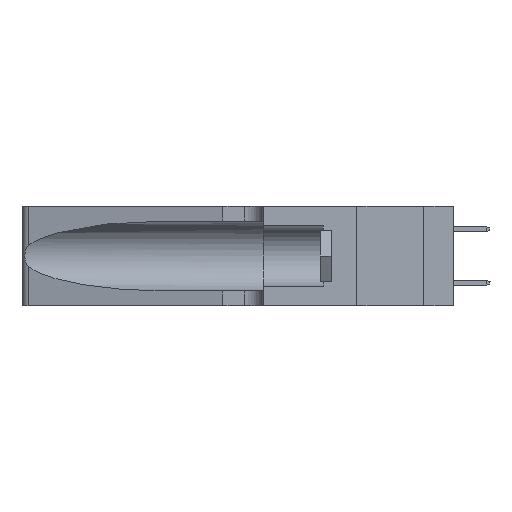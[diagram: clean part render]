
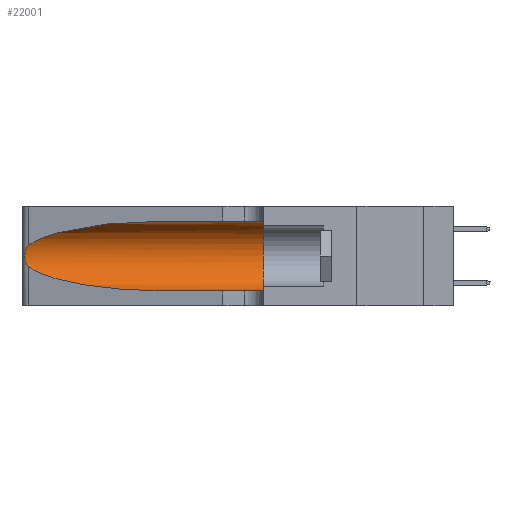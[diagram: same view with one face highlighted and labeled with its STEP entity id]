
A CAD part, left-side view. The second image highlights one B-rep face of the part: STEP entity #22001.
In plain terms, the highlighted cylindrical face has radius 3.308 mm (diameter 6.617 mm), a partial arc.
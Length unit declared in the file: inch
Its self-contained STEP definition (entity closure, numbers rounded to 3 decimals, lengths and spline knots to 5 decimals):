
#68 =( BOUNDED_CURVE ( )  B_SPLINE_CURVE ( 3, ( #24238, #24085, #4508, #12132 ),
 .UNSPECIFIED., .F., .T. ) 
 B_SPLINE_CURVE_WITH_KNOTS ( ( 4, 4 ),
 ( 3.44316, 4.71239 ),
 .UNSPECIFIED. ) 
 CURVE ( )  GEOMETRIC_REPRESENTATION_ITEM ( )  RATIONAL_B_SPLINE_CURVE ( ( 1., 0.87, 0.87, 1. ) ) 
 REPRESENTATION_ITEM ( '' )  );
#408 = VERTEX_POINT ( 'NONE', #10371 ) ;
#1938 = LINE ( 'NONE', #28831, #18233 ) ;
#2005 = CARTESIAN_POINT ( 'NONE',  ( 0.26075, 1.23896, 0.19203 ) ) ;
#2246 = EDGE_CURVE ( 'NONE', #24815, #27733, #1938, .T. ) ;
#2313 = CARTESIAN_POINT ( 'NONE',  ( 0.26075, 1.23896, 0.178 ) ) ;
#2868 = CIRCLE ( 'NONE', #19618, 0.13025 ) ;
#2886 = CARTESIAN_POINT ( 'NONE',  ( 0.2373, 1.15595, 0.28018 ) ) ;
#2993 = DIRECTION ( 'NONE',  ( 0., 1., 0. ) ) ;
#3141 =( BOUNDED_CURVE ( )  B_SPLINE_CURVE ( 3, ( #15765, #13228, #2886, #17662 ),
 .UNSPECIFIED., .F., .T. ) 
 B_SPLINE_CURVE_WITH_KNOTS ( ( 4, 4 ),
 ( 1.5708, 2.84003 ),
 .UNSPECIFIED. ) 
 CURVE ( )  GEOMETRIC_REPRESENTATION_ITEM ( )  RATIONAL_B_SPLINE_CURVE ( ( 1., 0.87, 0.87, 1. ) ) 
 REPRESENTATION_ITEM ( '' )  );
#3191 = CARTESIAN_POINT ( 'NONE',  ( 0.1305, 1.61858, 0.185 ) ) ;
#3346 = DIRECTION ( 'NONE',  ( 0., -1., 0. ) ) ;
#3574 = EDGE_LOOP ( 'NONE', ( #28299, #9650, #9836, #11445, #8035, #4098 ) ) ;
#4092 = CARTESIAN_POINT ( 'NONE',  ( 0.25787, 1.23484, 0.2124 ) ) ;
#4098 = ORIENTED_EDGE ( 'NONE', *, *, #2246, .F. ) ;
#4508 = CARTESIAN_POINT ( 'NONE',  ( 0.18966, 0.96281, 0.05475 ) ) ;
#4553 = CARTESIAN_POINT ( 'NONE',  ( 0.26017, 1.23833, 0.17102 ) ) ;
#5587 = CARTESIAN_POINT ( 'NONE',  ( 0.25487, 1.22718, 0.22369 ) ) ;
#6164 = CARTESIAN_POINT ( 'NONE',  ( 0.25487, 1.22718, 0.22369 ) ) ;
#7413 = AXIS2_PLACEMENT_3D ( 'NONE', #3191, #17329, #20341 ) ;
#7646 = CYLINDRICAL_SURFACE ( 'NONE', #7413, 0.13025 ) ;
#8035 = ORIENTED_EDGE ( 'NONE', *, *, #8123, .F. ) ;
#8123 = EDGE_CURVE ( 'NONE', #27733, #22074, #2868, .T. ) ;
#9606 = CARTESIAN_POINT ( 'NONE',  ( 0.25856, 1.23593, 0.16098 ) ) ;
#9640 = EDGE_CURVE ( 'NONE', #14535, #408, #68, .T. ) ;
#9650 = ORIENTED_EDGE ( 'NONE', *, *, #21707, .T. ) ;
#9657 = CARTESIAN_POINT ( 'NONE',  ( 0.1305, 0.35, 0.185 ) ) ;
#9673 = B_SPLINE_CURVE_WITH_KNOTS ( 'NONE', 3,
 ( #6164, #13802, #19027, #4092, #24127, #16796, #2005, #2313, #4553, #9606, #16496, #11391, #18712, #23791 ),
 .UNSPECIFIED., .F., .F.,
 ( 4, 2, 2, 2, 2, 2, 4 ),
 ( 0., 0.00027, 0.00053, 0.00107, 0.0016, 0.00187, 0.00214 ),
 .UNSPECIFIED. ) ;
#9836 = ORIENTED_EDGE ( 'NONE', *, *, #9640, .T. ) ;
#10371 = CARTESIAN_POINT ( 'NONE',  ( 0.1305, 0.72297, 0.05475 ) ) ;
#11391 = CARTESIAN_POINT ( 'NONE',  ( 0.25639, 1.23186, 0.15144 ) ) ;
#11445 = ORIENTED_EDGE ( 'NONE', *, *, #14961, .T. ) ;
#12132 = CARTESIAN_POINT ( 'NONE',  ( 0.1305, 0.72297, 0.05475 ) ) ;
#13228 = CARTESIAN_POINT ( 'NONE',  ( 0.18966, 0.96281, 0.31525 ) ) ;
#13802 = CARTESIAN_POINT ( 'NONE',  ( 0.25555, 1.22994, 0.2215 ) ) ;
#14535 = VERTEX_POINT ( 'NONE', #15484 ) ;
#14961 = EDGE_CURVE ( 'NONE', #408, #22074, #15446, .T. ) ;
#15446 = LINE ( 'NONE', #28024, #30075 ) ;
#15484 = CARTESIAN_POINT ( 'NONE',  ( 0.25487, 1.22718, 0.14631 ) ) ;
#15765 = CARTESIAN_POINT ( 'NONE',  ( 0.1305, 0.72297, 0.31525 ) ) ;
#16496 = CARTESIAN_POINT ( 'NONE',  ( 0.25789, 1.23486, 0.15765 ) ) ;
#16796 = CARTESIAN_POINT ( 'NONE',  ( 0.26018, 1.23835, 0.19895 ) ) ;
#17329 = DIRECTION ( 'NONE',  ( 0., -1., 0. ) ) ;
#17662 = CARTESIAN_POINT ( 'NONE',  ( 0.25487, 1.22718, 0.22369 ) ) ;
#18233 = VECTOR ( 'NONE', #31103, 39.37008 ) ;
#18712 = CARTESIAN_POINT ( 'NONE',  ( 0.25555, 1.22993, 0.14849 ) ) ;
#19027 = CARTESIAN_POINT ( 'NONE',  ( 0.25639, 1.23184, 0.21858 ) ) ;
#19618 = AXIS2_PLACEMENT_3D ( 'NONE', #9657, #2993, #29264 ) ;
#20341 = DIRECTION ( 'NONE',  ( 0., 0., -1. ) ) ;
#20917 = VERTEX_POINT ( 'NONE', #5587 ) ;
#21707 = EDGE_CURVE ( 'NONE', #20917, #14535, #9673, .T. ) ;
#22001 = ADVANCED_FACE ( 'NONE', ( #25005 ), #7646, .F. ) ;
#22074 = VERTEX_POINT ( 'NONE', #25465 ) ;
#23791 = CARTESIAN_POINT ( 'NONE',  ( 0.25487, 1.22718, 0.14631 ) ) ;
#24085 = CARTESIAN_POINT ( 'NONE',  ( 0.2373, 1.15595, 0.08982 ) ) ;
#24127 = CARTESIAN_POINT ( 'NONE',  ( 0.25854, 1.2359, 0.20912 ) ) ;
#24238 = CARTESIAN_POINT ( 'NONE',  ( 0.25487, 1.22718, 0.14631 ) ) ;
#24815 = VERTEX_POINT ( 'NONE', #30957 ) ;
#25005 = FACE_OUTER_BOUND ( 'NONE', #3574, .T. ) ;
#25465 = CARTESIAN_POINT ( 'NONE',  ( 0.1305, 0.35, 0.05475 ) ) ;
#27733 = VERTEX_POINT ( 'NONE', #29083 ) ;
#28024 = CARTESIAN_POINT ( 'NONE',  ( 0.1305, 1.61858, 0.05475 ) ) ;
#28299 = ORIENTED_EDGE ( 'NONE', *, *, #29515, .T. ) ;
#28831 = CARTESIAN_POINT ( 'NONE',  ( 0.1305, 1.61858, 0.31525 ) ) ;
#29083 = CARTESIAN_POINT ( 'NONE',  ( 0.1305, 0.35, 0.31525 ) ) ;
#29264 = DIRECTION ( 'NONE',  ( 0., 0., 1. ) ) ;
#29515 = EDGE_CURVE ( 'NONE', #24815, #20917, #3141, .T. ) ;
#30075 = VECTOR ( 'NONE', #3346, 39.37008 ) ;
#30957 = CARTESIAN_POINT ( 'NONE',  ( 0.1305, 0.72297, 0.31525 ) ) ;
#31103 = DIRECTION ( 'NONE',  ( 0., -1., 0. ) ) ;
